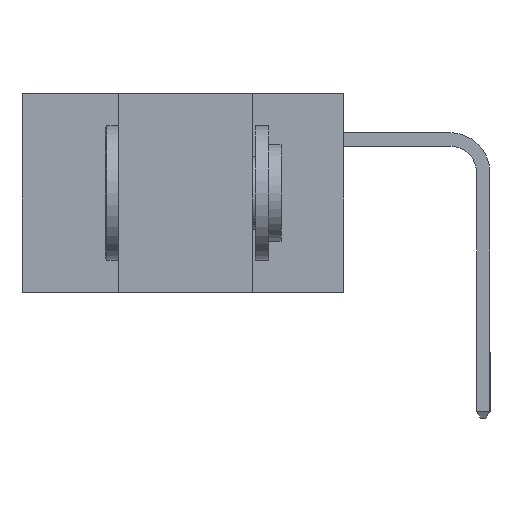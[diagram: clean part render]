
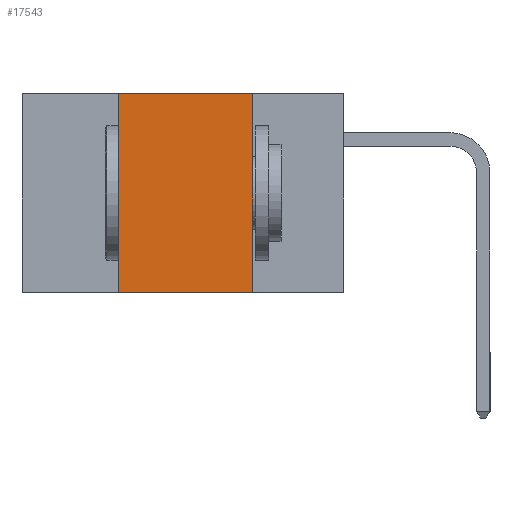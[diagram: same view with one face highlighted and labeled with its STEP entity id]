
A CAD part, left-side view. The second image highlights one B-rep face of the part: STEP entity #17543.
In plain terms, the highlighted planar face has unit normal (-1, 0, 0).
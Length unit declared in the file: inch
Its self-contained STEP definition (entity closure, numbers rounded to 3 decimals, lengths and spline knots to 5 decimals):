
#239 = DIRECTION ( 'NONE',  ( 0., -1., 0. ) ) ;
#538 = CARTESIAN_POINT ( 'NONE',  ( 0., 0.42, 0. ) ) ;
#1553 = PLANE ( 'NONE',  #9065 ) ;
#2352 = ORIENTED_EDGE ( 'NONE', *, *, #17748, .F. ) ;
#2998 = CARTESIAN_POINT ( 'NONE',  ( 0., 0.6, 0. ) ) ;
#3424 = DIRECTION ( 'NONE',  ( 0., 0., 1. ) ) ;
#4450 = DIRECTION ( 'NONE',  ( 1., 0., 0. ) ) ;
#4506 = EDGE_CURVE ( 'NONE', #9703, #16612, #9505, .T. ) ;
#5560 = CARTESIAN_POINT ( 'NONE',  ( 0., 0.17, -0.37 ) ) ;
#6077 = ORIENTED_EDGE ( 'NONE', *, *, #4506, .F. ) ;
#6084 = EDGE_CURVE ( 'NONE', #16612, #14767, #6723, .T. ) ;
#6269 = VECTOR ( 'NONE', #9655, 39.37008 ) ;
#6589 = FACE_OUTER_BOUND ( 'NONE', #11072, .T. ) ;
#6723 = LINE ( 'NONE', #10765, #6269 ) ;
#6807 = VECTOR ( 'NONE', #3424, 39.37008 ) ;
#7154 = EDGE_CURVE ( 'NONE', #13792, #14767, #17922, .T. ) ;
#7247 = LINE ( 'NONE', #538, #6807 ) ;
#7256 = ORIENTED_EDGE ( 'NONE', *, *, #7154, .T. ) ;
#9065 = AXIS2_PLACEMENT_3D ( 'NONE', #2998, #4450, #14516 ) ;
#9505 = LINE ( 'NONE', #10766, #16656 ) ;
#9655 = DIRECTION ( 'NONE',  ( 0., 0., -1. ) ) ;
#9703 = VERTEX_POINT ( 'NONE', #9853 ) ;
#9853 = CARTESIAN_POINT ( 'NONE',  ( 0., 0.42, 0. ) ) ;
#9879 = VECTOR ( 'NONE', #10278, 39.37008 ) ;
#10278 = DIRECTION ( 'NONE',  ( 0., -1., 0. ) ) ;
#10765 = CARTESIAN_POINT ( 'NONE',  ( 0., 0.17, 0. ) ) ;
#10766 = CARTESIAN_POINT ( 'NONE',  ( 0., 0.6, 0. ) ) ;
#11072 = EDGE_LOOP ( 'NONE', ( #17356, #6077, #2352, #7256 ) ) ;
#11419 = CARTESIAN_POINT ( 'NONE',  ( 0., 0.6, -0.37 ) ) ;
#13792 = VERTEX_POINT ( 'NONE', #14782 ) ;
#14516 = DIRECTION ( 'NONE',  ( 0., 0., -1. ) ) ;
#14767 = VERTEX_POINT ( 'NONE', #5560 ) ;
#14782 = CARTESIAN_POINT ( 'NONE',  ( 0., 0.42, -0.37 ) ) ;
#16612 = VERTEX_POINT ( 'NONE', #16660 ) ;
#16656 = VECTOR ( 'NONE', #239, 39.37008 ) ;
#16660 = CARTESIAN_POINT ( 'NONE',  ( 0., 0.17, 0. ) ) ;
#17356 = ORIENTED_EDGE ( 'NONE', *, *, #6084, .F. ) ;
#17543 = ADVANCED_FACE ( 'NONE', ( #6589 ), #1553, .F. ) ;
#17748 = EDGE_CURVE ( 'NONE', #13792, #9703, #7247, .T. ) ;
#17922 = LINE ( 'NONE', #11419, #9879 ) ;
